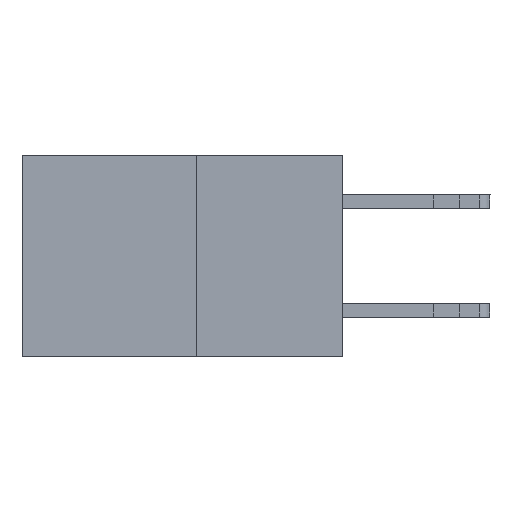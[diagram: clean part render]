
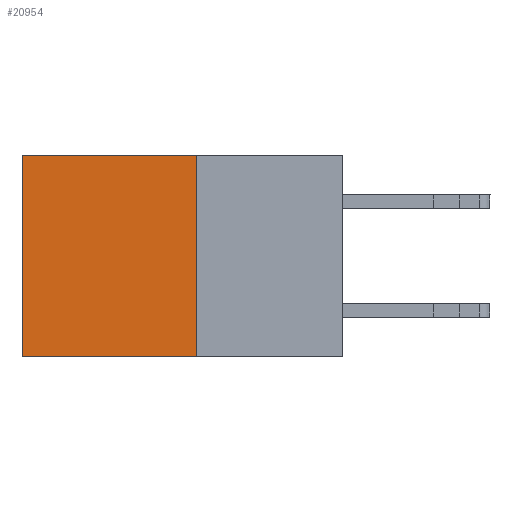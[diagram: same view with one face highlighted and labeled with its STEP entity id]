
A CAD part, left-side view. The second image highlights one B-rep face of the part: STEP entity #20954.
In plain terms, the highlighted planar face has unit normal (-1, 0, 0).
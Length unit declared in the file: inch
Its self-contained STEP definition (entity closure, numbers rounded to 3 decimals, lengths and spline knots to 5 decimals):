
#497 = DIRECTION ( 'NONE',  ( 0., 1., 0. ) ) ;
#949 = EDGE_CURVE ( 'NONE', #25912, #2423, #11158, .T. ) ;
#2423 = VERTEX_POINT ( 'NONE', #5477 ) ;
#2661 = EDGE_CURVE ( 'NONE', #8665, #11531, #23745, .T. ) ;
#2955 = CARTESIAN_POINT ( 'NONE',  ( 0.277, 0.27, -0.37 ) ) ;
#3227 = PLANE ( 'NONE',  #17271 ) ;
#3413 = EDGE_CURVE ( 'NONE', #11531, #2423, #7115, .T. ) ;
#5477 = CARTESIAN_POINT ( 'NONE',  ( 0.277, 0.59, -0.37 ) ) ;
#5604 = ORIENTED_EDGE ( 'NONE', *, *, #24093, .F. ) ;
#6836 = DIRECTION ( 'NONE',  ( 0., 0., -1. ) ) ;
#7115 = LINE ( 'NONE', #23603, #8763 ) ;
#7886 = DIRECTION ( 'NONE',  ( 0., 0., -1. ) ) ;
#8665 = VERTEX_POINT ( 'NONE', #25945 ) ;
#8763 = VECTOR ( 'NONE', #6836, 39.37008 ) ;
#9489 = ORIENTED_EDGE ( 'NONE', *, *, #949, .F. ) ;
#10748 = VECTOR ( 'NONE', #7886, 39.37008 ) ;
#10997 = CARTESIAN_POINT ( 'NONE',  ( 0.277, 0.27, 0. ) ) ;
#11019 = CARTESIAN_POINT ( 'NONE',  ( 0.277, 0.27, -0.37 ) ) ;
#11158 = LINE ( 'NONE', #11019, #21358 ) ;
#11531 = VERTEX_POINT ( 'NONE', #23378 ) ;
#11667 = DIRECTION ( 'NONE',  ( 0., 0., -1. ) ) ;
#11800 = DIRECTION ( 'NONE',  ( 1., 0., 0. ) ) ;
#11996 = CARTESIAN_POINT ( 'NONE',  ( 0.277, 0.27, -0.37 ) ) ;
#12519 = ORIENTED_EDGE ( 'NONE', *, *, #2661, .T. ) ;
#15825 = FACE_OUTER_BOUND ( 'NONE', #24494, .T. ) ;
#17271 = AXIS2_PLACEMENT_3D ( 'NONE', #2955, #11800, #11667 ) ;
#20954 = ADVANCED_FACE ( 'NONE', ( #15825 ), #3227, .F. ) ;
#21358 = VECTOR ( 'NONE', #497, 39.37008 ) ;
#21533 = DIRECTION ( 'NONE',  ( 0., 1., 0. ) ) ;
#22580 = CARTESIAN_POINT ( 'NONE',  ( 0.277, 0.27, -0.37 ) ) ;
#23373 = VECTOR ( 'NONE', #21533, 39.37008 ) ;
#23378 = CARTESIAN_POINT ( 'NONE',  ( 0.277, 0.59, 0. ) ) ;
#23603 = CARTESIAN_POINT ( 'NONE',  ( 0.277, 0.59, -0.37 ) ) ;
#23745 = LINE ( 'NONE', #10997, #23373 ) ;
#24093 = EDGE_CURVE ( 'NONE', #8665, #25912, #26461, .T. ) ;
#24494 = EDGE_LOOP ( 'NONE', ( #25134, #9489, #5604, #12519 ) ) ;
#25134 = ORIENTED_EDGE ( 'NONE', *, *, #3413, .T. ) ;
#25912 = VERTEX_POINT ( 'NONE', #11996 ) ;
#25945 = CARTESIAN_POINT ( 'NONE',  ( 0.277, 0.27, 0. ) ) ;
#26461 = LINE ( 'NONE', #22580, #10748 ) ;
